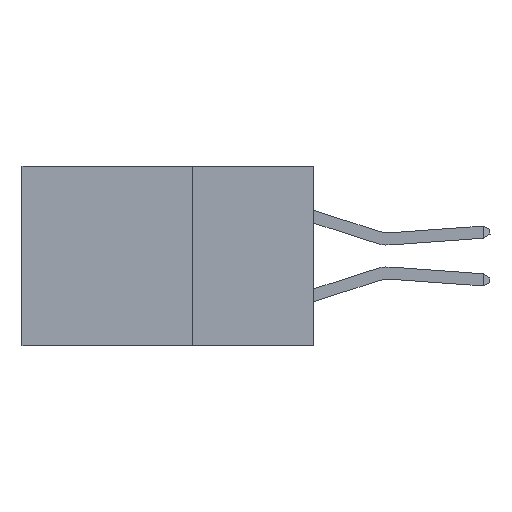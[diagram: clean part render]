
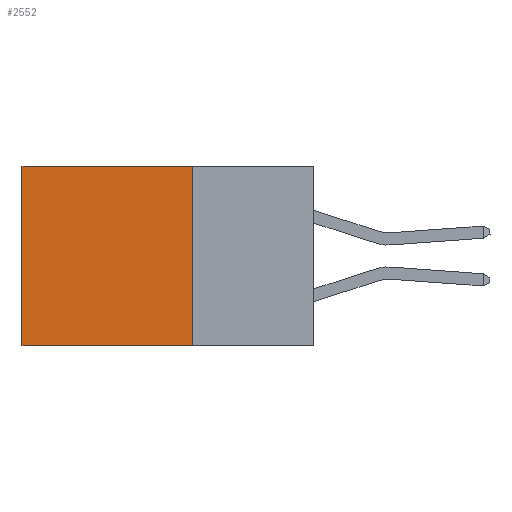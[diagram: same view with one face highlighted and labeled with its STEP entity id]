
A CAD part, left-side view. The second image highlights one B-rep face of the part: STEP entity #2552.
In plain terms, the highlighted planar face has unit normal (-1, 0, 0).
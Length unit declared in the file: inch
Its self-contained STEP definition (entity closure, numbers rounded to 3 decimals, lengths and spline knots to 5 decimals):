
#10 = AXIS2_PLACEMENT_3D ( 'NONE', #19915, #636, #5583 ) ;
#113 = EDGE_LOOP ( 'NONE', ( #6615, #15493, #20251, #8297 ) ) ;
#636 = DIRECTION ( 'NONE',  ( 1., 0., 0. ) ) ;
#680 = LINE ( 'NONE', #4531, #19618 ) ;
#704 = LINE ( 'NONE', #9970, #20125 ) ;
#1630 = VERTEX_POINT ( 'NONE', #11031 ) ;
#1743 = CARTESIAN_POINT ( 'NONE',  ( 0.2875, 0.25, -0.37 ) ) ;
#2118 = EDGE_CURVE ( 'NONE', #1630, #6817, #680, .T. ) ;
#2552 = ADVANCED_FACE ( 'NONE', ( #7687 ), #18132, .F. ) ;
#4531 = CARTESIAN_POINT ( 'NONE',  ( 0.2875, 0.25, 0. ) ) ;
#5583 = DIRECTION ( 'NONE',  ( 0., 0., -1. ) ) ;
#6163 = CARTESIAN_POINT ( 'NONE',  ( 0.2875, 0.6, 0. ) ) ;
#6358 = CARTESIAN_POINT ( 'NONE',  ( 0.2875, 0.6, 0. ) ) ;
#6615 = ORIENTED_EDGE ( 'NONE', *, *, #10448, .T. ) ;
#6817 = VERTEX_POINT ( 'NONE', #6358 ) ;
#7687 = FACE_OUTER_BOUND ( 'NONE', #113, .T. ) ;
#8297 = ORIENTED_EDGE ( 'NONE', *, *, #2118, .T. ) ;
#9660 = EDGE_CURVE ( 'NONE', #15543, #16741, #11436, .T. ) ;
#9970 = CARTESIAN_POINT ( 'NONE',  ( 0.2875, 0.25, 0. ) ) ;
#10448 = EDGE_CURVE ( 'NONE', #6817, #16741, #14682, .T. ) ;
#10548 = CARTESIAN_POINT ( 'NONE',  ( 0.2875, 0.25, -0.37 ) ) ;
#10616 = EDGE_CURVE ( 'NONE', #1630, #15543, #704, .T. ) ;
#10773 = CARTESIAN_POINT ( 'NONE',  ( 0.2875, 0.6, -0.37 ) ) ;
#10807 = DIRECTION ( 'NONE',  ( 0., 1., 0. ) ) ;
#11031 = CARTESIAN_POINT ( 'NONE',  ( 0.2875, 0.25, 0. ) ) ;
#11436 = LINE ( 'NONE', #1743, #13674 ) ;
#13674 = VECTOR ( 'NONE', #15946, 39.37008 ) ;
#14147 = VECTOR ( 'NONE', #14163, 39.37008 ) ;
#14163 = DIRECTION ( 'NONE',  ( 0., 0., -1. ) ) ;
#14682 = LINE ( 'NONE', #6163, #14147 ) ;
#14766 = DIRECTION ( 'NONE',  ( 0., 0., -1. ) ) ;
#15493 = ORIENTED_EDGE ( 'NONE', *, *, #9660, .F. ) ;
#15543 = VERTEX_POINT ( 'NONE', #10548 ) ;
#15946 = DIRECTION ( 'NONE',  ( 0., 1., 0. ) ) ;
#16741 = VERTEX_POINT ( 'NONE', #10773 ) ;
#18132 = PLANE ( 'NONE',  #10 ) ;
#19618 = VECTOR ( 'NONE', #10807, 39.37008 ) ;
#19915 = CARTESIAN_POINT ( 'NONE',  ( 0.2875, 0.25, 0. ) ) ;
#20125 = VECTOR ( 'NONE', #14766, 39.37008 ) ;
#20251 = ORIENTED_EDGE ( 'NONE', *, *, #10616, .F. ) ;
